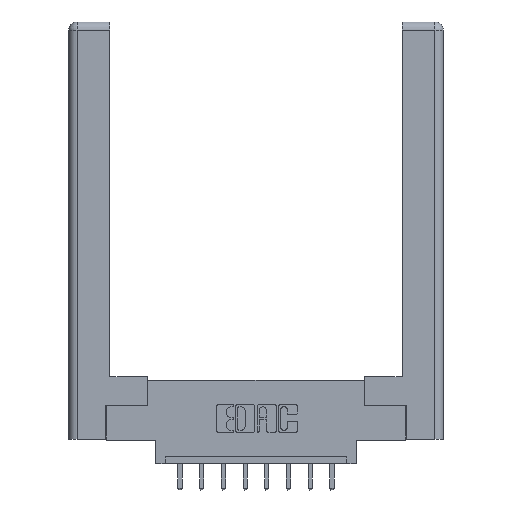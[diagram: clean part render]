
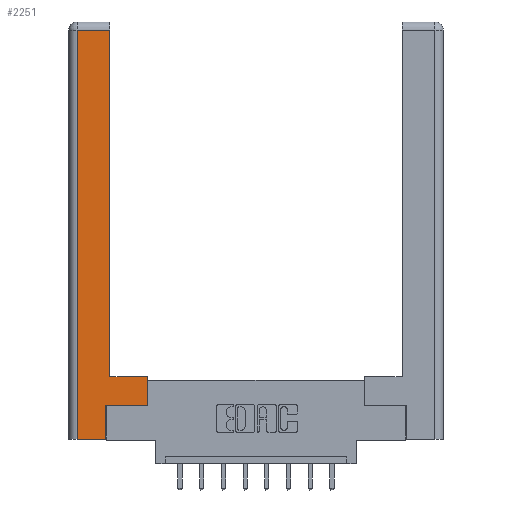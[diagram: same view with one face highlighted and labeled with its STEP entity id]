
A CAD part, top view. The second image highlights one B-rep face of the part: STEP entity #2251.
In plain terms, the highlighted planar face has unit normal (0, 0, 1).
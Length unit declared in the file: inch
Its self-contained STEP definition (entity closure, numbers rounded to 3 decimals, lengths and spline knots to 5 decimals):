
#98 = VECTOR ( 'NONE', #1951, 39.37008 ) ;
#881 = CARTESIAN_POINT ( 'NONE',  ( 0.565, 0.45, 0. ) ) ;
#1101 = VECTOR ( 'NONE', #13167, 39.37008 ) ;
#1322 = EDGE_CURVE ( 'NONE', #7040, #7312, #8576, .T. ) ;
#1368 = ORIENTED_EDGE ( 'NONE', *, *, #9918, .T. ) ;
#1465 = EDGE_CURVE ( 'NONE', #5671, #2862, #4567, .T. ) ;
#1823 = DIRECTION ( 'NONE',  ( 1., 0., 0. ) ) ;
#1868 = DIRECTION ( 'NONE',  ( 0., 1., 0. ) ) ;
#1951 = DIRECTION ( 'NONE',  ( 0., 1., 0. ) ) ;
#1966 = ORIENTED_EDGE ( 'NONE', *, *, #3109, .T. ) ;
#2208 = ORIENTED_EDGE ( 'NONE', *, *, #10346, .T. ) ;
#2251 = ADVANCED_FACE ( 'NONE', ( #9775 ), #11206, .F. ) ;
#2384 = DIRECTION ( 'NONE',  ( -1., 0., 0. ) ) ;
#2862 = VERTEX_POINT ( 'NONE', #2958 ) ;
#2958 = CARTESIAN_POINT ( 'NONE',  ( 0.0615, 0., 0. ) ) ;
#3109 = EDGE_CURVE ( 'NONE', #13080, #8488, #5612, .T. ) ;
#3121 = DIRECTION ( 'NONE',  ( -1., 0., 0. ) ) ;
#3768 = CARTESIAN_POINT ( 'NONE',  ( 0.0615, 0., 0. ) ) ;
#4101 = LINE ( 'NONE', #10110, #9670 ) ;
#4209 = EDGE_CURVE ( 'NONE', #6431, #13080, #12322, .T. ) ;
#4567 = LINE ( 'NONE', #3768, #12099 ) ;
#4822 = EDGE_CURVE ( 'NONE', #7312, #7119, #12767, .T. ) ;
#5028 = CARTESIAN_POINT ( 'NONE',  ( 0.565, 0.245, 0. ) ) ;
#5210 = LINE ( 'NONE', #12618, #13199 ) ;
#5319 = CARTESIAN_POINT ( 'NONE',  ( 0.295, 0.45, 0. ) ) ;
#5513 = ORIENTED_EDGE ( 'NONE', *, *, #1465, .T. ) ;
#5612 = LINE ( 'NONE', #6901, #9928 ) ;
#5671 = VERTEX_POINT ( 'NONE', #8133 ) ;
#5680 = CARTESIAN_POINT ( 'NONE',  ( 0.265, 0., 0. ) ) ;
#5701 = AXIS2_PLACEMENT_3D ( 'NONE', #13205, #13251, #3121 ) ;
#5848 = VECTOR ( 'NONE', #1868, 39.37008 ) ;
#6431 = VERTEX_POINT ( 'NONE', #11680 ) ;
#6483 = DIRECTION ( 'NONE',  ( -1., 0., 0. ) ) ;
#6901 = CARTESIAN_POINT ( 'NONE',  ( 0.295, 3., 0. ) ) ;
#7040 = VERTEX_POINT ( 'NONE', #5680 ) ;
#7119 = VERTEX_POINT ( 'NONE', #10122 ) ;
#7261 = ORIENTED_EDGE ( 'NONE', *, *, #1322, .T. ) ;
#7312 = VERTEX_POINT ( 'NONE', #12360 ) ;
#7350 = DIRECTION ( 'NONE',  ( 0., 1., 0. ) ) ;
#8133 = CARTESIAN_POINT ( 'NONE',  ( 0.0615, 2.94, 0. ) ) ;
#8458 = VECTOR ( 'NONE', #2384, 39.37008 ) ;
#8488 = VERTEX_POINT ( 'NONE', #8999 ) ;
#8576 = LINE ( 'NONE', #9944, #5848 ) ;
#8999 = CARTESIAN_POINT ( 'NONE',  ( 0.295, 2.94, 0. ) ) ;
#9670 = VECTOR ( 'NONE', #1823, 39.37008 ) ;
#9775 = FACE_OUTER_BOUND ( 'NONE', #12616, .T. ) ;
#9918 = EDGE_CURVE ( 'NONE', #2862, #7040, #4101, .T. ) ;
#9928 = VECTOR ( 'NONE', #7350, 39.37008 ) ;
#9944 = CARTESIAN_POINT ( 'NONE',  ( 0.265, 0.245, 0. ) ) ;
#10110 = CARTESIAN_POINT ( 'NONE',  ( 0.265, 0., 0. ) ) ;
#10122 = CARTESIAN_POINT ( 'NONE',  ( 0.565, 0.245, 0. ) ) ;
#10327 = EDGE_CURVE ( 'NONE', #7119, #6431, #12079, .T. ) ;
#10346 = EDGE_CURVE ( 'NONE', #8488, #5671, #5210, .T. ) ;
#10624 = CARTESIAN_POINT ( 'NONE',  ( 0.295, 0.45, 0. ) ) ;
#10777 = ORIENTED_EDGE ( 'NONE', *, *, #4822, .T. ) ;
#10924 = DIRECTION ( 'NONE',  ( 0., -1., 0. ) ) ;
#11002 = ORIENTED_EDGE ( 'NONE', *, *, #4209, .T. ) ;
#11206 = PLANE ( 'NONE',  #5701 ) ;
#11680 = CARTESIAN_POINT ( 'NONE',  ( 0.565, 0.45, 0. ) ) ;
#12079 = LINE ( 'NONE', #881, #98 ) ;
#12099 = VECTOR ( 'NONE', #10924, 39.37008 ) ;
#12322 = LINE ( 'NONE', #10624, #8458 ) ;
#12360 = CARTESIAN_POINT ( 'NONE',  ( 0.265, 0.245, 0. ) ) ;
#12616 = EDGE_LOOP ( 'NONE', ( #1966, #2208, #5513, #1368, #7261, #10777, #12646, #11002 ) ) ;
#12618 = CARTESIAN_POINT ( 'NONE',  ( 0.0615, 2.94, 0. ) ) ;
#12646 = ORIENTED_EDGE ( 'NONE', *, *, #10327, .T. ) ;
#12767 = LINE ( 'NONE', #5028, #1101 ) ;
#13080 = VERTEX_POINT ( 'NONE', #5319 ) ;
#13167 = DIRECTION ( 'NONE',  ( 1., 0., 0. ) ) ;
#13199 = VECTOR ( 'NONE', #6483, 39.37008 ) ;
#13205 = CARTESIAN_POINT ( 'NONE',  ( 0., 0., 0. ) ) ;
#13251 = DIRECTION ( 'NONE',  ( 0., 0., -1. ) ) ;
